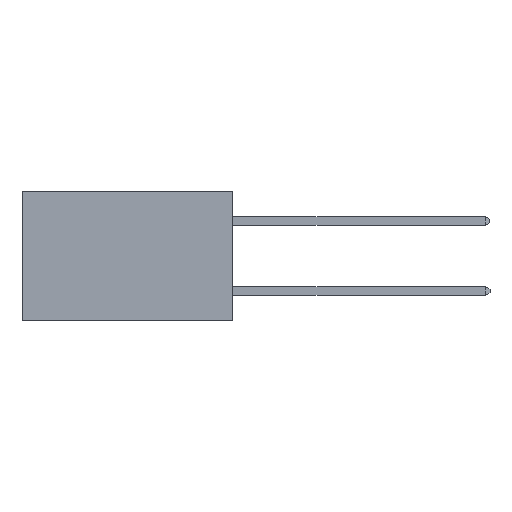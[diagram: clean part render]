
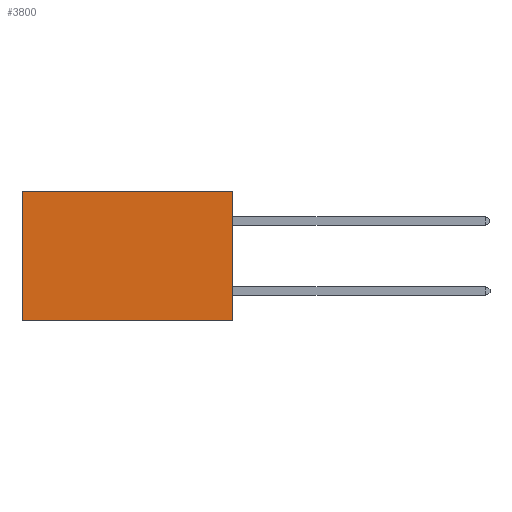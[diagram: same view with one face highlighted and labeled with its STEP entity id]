
A CAD part, left-side view. The second image highlights one B-rep face of the part: STEP entity #3800.
In plain terms, the highlighted planar face has unit normal (-1, 0, 0).
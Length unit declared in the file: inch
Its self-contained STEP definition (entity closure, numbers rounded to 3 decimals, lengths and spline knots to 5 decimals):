
#53 = VECTOR ( 'NONE', #3431, 39.37008 ) ;
#401 = VECTOR ( 'NONE', #5259, 39.37008 ) ;
#2565 = FACE_OUTER_BOUND ( 'NONE', #7521, .T. ) ;
#2599 = VERTEX_POINT ( 'NONE', #13060 ) ;
#3431 = DIRECTION ( 'NONE',  ( 0., 1., 0. ) ) ;
#3793 = CARTESIAN_POINT ( 'NONE',  ( 0.2875, 0.6, 0. ) ) ;
#3800 = ADVANCED_FACE ( 'NONE', ( #2565 ), #6232, .F. ) ;
#5259 = DIRECTION ( 'NONE',  ( 0., 1., 0. ) ) ;
#5940 = AXIS2_PLACEMENT_3D ( 'NONE', #9158, #9184, #14543 ) ;
#5987 = EDGE_CURVE ( 'NONE', #13743, #2599, #11367, .T. ) ;
#6232 = PLANE ( 'NONE',  #5940 ) ;
#6262 = ORIENTED_EDGE ( 'NONE', *, *, #8909, .F. ) ;
#6756 = CARTESIAN_POINT ( 'NONE',  ( 0.2875, 0., 0. ) ) ;
#7521 = EDGE_LOOP ( 'NONE', ( #11919, #6262, #12562, #9443 ) ) ;
#8168 = CARTESIAN_POINT ( 'NONE',  ( 0.2875, 0.6, -0.37 ) ) ;
#8909 = EDGE_CURVE ( 'NONE', #15342, #14225, #10972, .T. ) ;
#9035 = VECTOR ( 'NONE', #9541, 39.37008 ) ;
#9081 = EDGE_CURVE ( 'NONE', #2599, #14225, #15261, .T. ) ;
#9158 = CARTESIAN_POINT ( 'NONE',  ( 0.2875, 0., 0. ) ) ;
#9184 = DIRECTION ( 'NONE',  ( 1., 0., 0. ) ) ;
#9443 = ORIENTED_EDGE ( 'NONE', *, *, #5987, .T. ) ;
#9541 = DIRECTION ( 'NONE',  ( 0., 0., -1. ) ) ;
#10972 = LINE ( 'NONE', #17168, #53 ) ;
#11367 = LINE ( 'NONE', #12072, #401 ) ;
#11620 = VECTOR ( 'NONE', #16214, 39.37008 ) ;
#11752 = CARTESIAN_POINT ( 'NONE',  ( 0.2875, 0., -0.37 ) ) ;
#11919 = ORIENTED_EDGE ( 'NONE', *, *, #9081, .T. ) ;
#12072 = CARTESIAN_POINT ( 'NONE',  ( 0.2875, 0., 0. ) ) ;
#12562 = ORIENTED_EDGE ( 'NONE', *, *, #14227, .F. ) ;
#13060 = CARTESIAN_POINT ( 'NONE',  ( 0.2875, 0.6, 0. ) ) ;
#13067 = LINE ( 'NONE', #6756, #9035 ) ;
#13586 = CARTESIAN_POINT ( 'NONE',  ( 0.2875, 0., 0. ) ) ;
#13743 = VERTEX_POINT ( 'NONE', #13586 ) ;
#14225 = VERTEX_POINT ( 'NONE', #8168 ) ;
#14227 = EDGE_CURVE ( 'NONE', #13743, #15342, #13067, .T. ) ;
#14543 = DIRECTION ( 'NONE',  ( 0., 0., -1. ) ) ;
#15261 = LINE ( 'NONE', #3793, #11620 ) ;
#15342 = VERTEX_POINT ( 'NONE', #11752 ) ;
#16214 = DIRECTION ( 'NONE',  ( 0., 0., -1. ) ) ;
#17168 = CARTESIAN_POINT ( 'NONE',  ( 0.2875, 0., -0.37 ) ) ;
